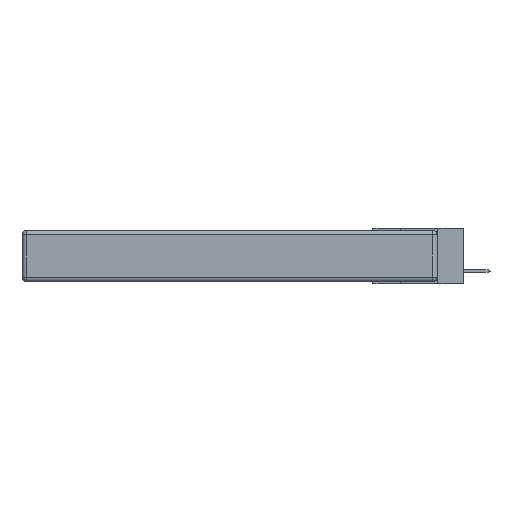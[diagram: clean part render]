
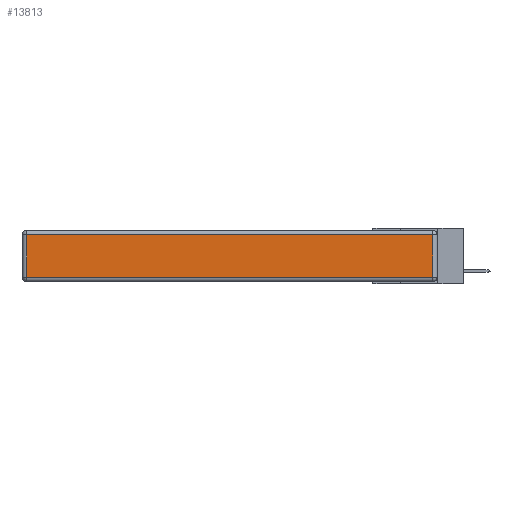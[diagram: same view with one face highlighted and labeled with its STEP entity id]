
A CAD part, left-side view. The second image highlights one B-rep face of the part: STEP entity #13813.
In plain terms, the highlighted planar face has unit normal (-1, 0, 0).
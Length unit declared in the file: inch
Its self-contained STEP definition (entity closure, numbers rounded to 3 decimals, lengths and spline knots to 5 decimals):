
#733 = LINE ( 'NONE', #4460, #8200 ) ;
#764 = VERTEX_POINT ( 'NONE', #14351 ) ;
#1033 = LINE ( 'NONE', #5162, #11311 ) ;
#1058 = VECTOR ( 'NONE', #14119, 39.37008 ) ;
#1380 = CARTESIAN_POINT ( 'NONE',  ( 0., 2.72, -0.343 ) ) ;
#2586 = CARTESIAN_POINT ( 'NONE',  ( 0., 0.03, -0.343 ) ) ;
#3202 = DIRECTION ( 'NONE',  ( 0., 0., 1. ) ) ;
#3720 = AXIS2_PLACEMENT_3D ( 'NONE', #8297, #12929, #3202 ) ;
#4460 = CARTESIAN_POINT ( 'NONE',  ( 0., 0., -0.313 ) ) ;
#4810 = PLANE ( 'NONE',  #3720 ) ;
#5162 = CARTESIAN_POINT ( 'NONE',  ( 0., 2.75, -0.03 ) ) ;
#5537 = EDGE_CURVE ( 'NONE', #16597, #764, #17116, .T. ) ;
#5905 = CARTESIAN_POINT ( 'NONE',  ( 0., 2.72, -0.03 ) ) ;
#6111 = ORIENTED_EDGE ( 'NONE', *, *, #16647, .T. ) ;
#7580 = VERTEX_POINT ( 'NONE', #14997 ) ;
#7727 = EDGE_CURVE ( 'NONE', #13471, #16597, #1033, .T. ) ;
#8200 = VECTOR ( 'NONE', #17674, 39.37008 ) ;
#8297 = CARTESIAN_POINT ( 'NONE',  ( 0., 0., -0.343 ) ) ;
#8684 = CARTESIAN_POINT ( 'NONE',  ( 0., 0.03, -0.03 ) ) ;
#9252 = ORIENTED_EDGE ( 'NONE', *, *, #7727, .T. ) ;
#9364 = ORIENTED_EDGE ( 'NONE', *, *, #5537, .T. ) ;
#10008 = DIRECTION ( 'NONE',  ( 0., 1., 0. ) ) ;
#10484 = EDGE_LOOP ( 'NONE', ( #17871, #6111, #9252, #9364 ) ) ;
#11311 = VECTOR ( 'NONE', #10008, 39.37008 ) ;
#11537 = FACE_OUTER_BOUND ( 'NONE', #10484, .T. ) ;
#12707 = DIRECTION ( 'NONE',  ( 0., 0., -1. ) ) ;
#12929 = DIRECTION ( 'NONE',  ( -1., 0., 0. ) ) ;
#13471 = VERTEX_POINT ( 'NONE', #8684 ) ;
#13813 = ADVANCED_FACE ( 'NONE', ( #11537 ), #4810, .T. ) ;
#14119 = DIRECTION ( 'NONE',  ( 0., 0., 1. ) ) ;
#14351 = CARTESIAN_POINT ( 'NONE',  ( 0., 2.72, -0.313 ) ) ;
#14997 = CARTESIAN_POINT ( 'NONE',  ( 0., 0.03, -0.313 ) ) ;
#16597 = VERTEX_POINT ( 'NONE', #5905 ) ;
#16647 = EDGE_CURVE ( 'NONE', #7580, #13471, #19343, .T. ) ;
#17116 = LINE ( 'NONE', #1380, #17630 ) ;
#17630 = VECTOR ( 'NONE', #12707, 39.37008 ) ;
#17674 = DIRECTION ( 'NONE',  ( 0., -1., 0. ) ) ;
#17871 = ORIENTED_EDGE ( 'NONE', *, *, #18828, .T. ) ;
#18828 = EDGE_CURVE ( 'NONE', #764, #7580, #733, .T. ) ;
#19343 = LINE ( 'NONE', #2586, #1058 ) ;
